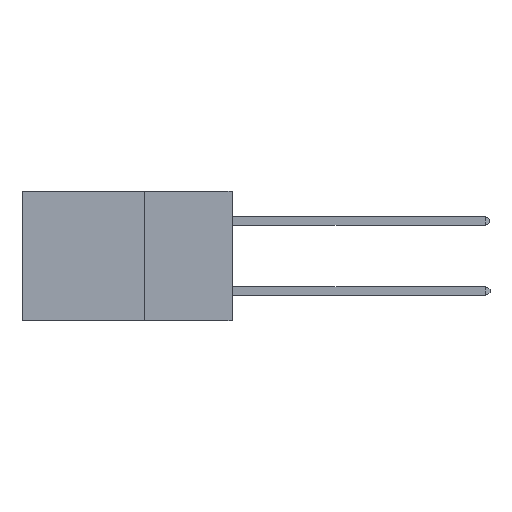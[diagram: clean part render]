
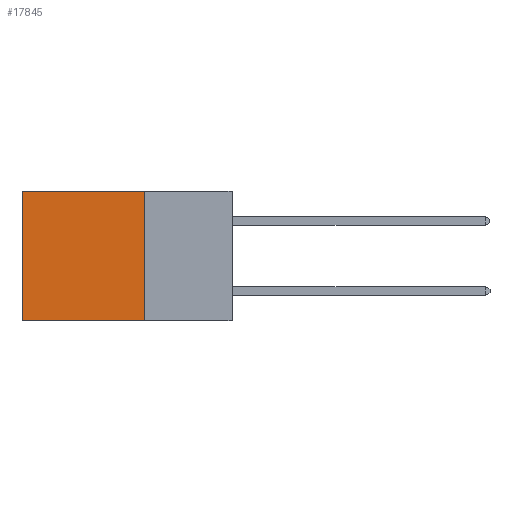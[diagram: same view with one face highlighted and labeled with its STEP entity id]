
A CAD part, left-side view. The second image highlights one B-rep face of the part: STEP entity #17845.
In plain terms, the highlighted planar face has unit normal (-1, 0, 0).
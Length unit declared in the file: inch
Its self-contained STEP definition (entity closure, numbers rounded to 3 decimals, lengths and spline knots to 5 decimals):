
#443 = DIRECTION ( 'NONE',  ( 0., 1., 0. ) ) ;
#726 = CARTESIAN_POINT ( 'NONE',  ( 0.2875, 0.6, -0.37 ) ) ;
#1099 = VERTEX_POINT ( 'NONE', #726 ) ;
#1147 = DIRECTION ( 'NONE',  ( 0., 0., -1. ) ) ;
#1642 = EDGE_CURVE ( 'NONE', #9766, #1099, #8186, .T. ) ;
#1838 = LINE ( 'NONE', #17591, #9119 ) ;
#2035 = AXIS2_PLACEMENT_3D ( 'NONE', #9984, #11520, #2271 ) ;
#2271 = DIRECTION ( 'NONE',  ( 0., 0., -1. ) ) ;
#2521 = EDGE_CURVE ( 'NONE', #4523, #9766, #1838, .T. ) ;
#4523 = VERTEX_POINT ( 'NONE', #10197 ) ;
#4609 = VECTOR ( 'NONE', #443, 39.37008 ) ;
#4986 = LINE ( 'NONE', #19347, #9068 ) ;
#5278 = EDGE_CURVE ( 'NONE', #5362, #1099, #4986, .T. ) ;
#5317 = VECTOR ( 'NONE', #14966, 39.37008 ) ;
#5362 = VERTEX_POINT ( 'NONE', #7553 ) ;
#5846 = FACE_OUTER_BOUND ( 'NONE', #7927, .T. ) ;
#7553 = CARTESIAN_POINT ( 'NONE',  ( 0.2875, 0.6, 0. ) ) ;
#7927 = EDGE_LOOP ( 'NONE', ( #12817, #12884, #12980, #13211 ) ) ;
#8186 = LINE ( 'NONE', #9727, #4609 ) ;
#9068 = VECTOR ( 'NONE', #1147, 39.37008 ) ;
#9119 = VECTOR ( 'NONE', #11652, 39.37008 ) ;
#9509 = EDGE_CURVE ( 'NONE', #4523, #5362, #17397, .T. ) ;
#9727 = CARTESIAN_POINT ( 'NONE',  ( 0.2875, 0.25, -0.37 ) ) ;
#9766 = VERTEX_POINT ( 'NONE', #15391 ) ;
#9984 = CARTESIAN_POINT ( 'NONE',  ( 0.2875, 0.25, 0. ) ) ;
#10197 = CARTESIAN_POINT ( 'NONE',  ( 0.2875, 0.25, 0. ) ) ;
#11520 = DIRECTION ( 'NONE',  ( 1., 0., 0. ) ) ;
#11652 = DIRECTION ( 'NONE',  ( 0., 0., -1. ) ) ;
#12817 = ORIENTED_EDGE ( 'NONE', *, *, #5278, .T. ) ;
#12884 = ORIENTED_EDGE ( 'NONE', *, *, #1642, .F. ) ;
#12980 = ORIENTED_EDGE ( 'NONE', *, *, #2521, .F. ) ;
#13211 = ORIENTED_EDGE ( 'NONE', *, *, #9509, .T. ) ;
#13450 = CARTESIAN_POINT ( 'NONE',  ( 0.2875, 0.25, 0. ) ) ;
#14966 = DIRECTION ( 'NONE',  ( 0., 1., 0. ) ) ;
#15391 = CARTESIAN_POINT ( 'NONE',  ( 0.2875, 0.25, -0.37 ) ) ;
#17397 = LINE ( 'NONE', #13450, #5317 ) ;
#17591 = CARTESIAN_POINT ( 'NONE',  ( 0.2875, 0.25, 0. ) ) ;
#17845 = ADVANCED_FACE ( 'NONE', ( #5846 ), #18926, .F. ) ;
#18926 = PLANE ( 'NONE',  #2035 ) ;
#19347 = CARTESIAN_POINT ( 'NONE',  ( 0.2875, 0.6, 0. ) ) ;
